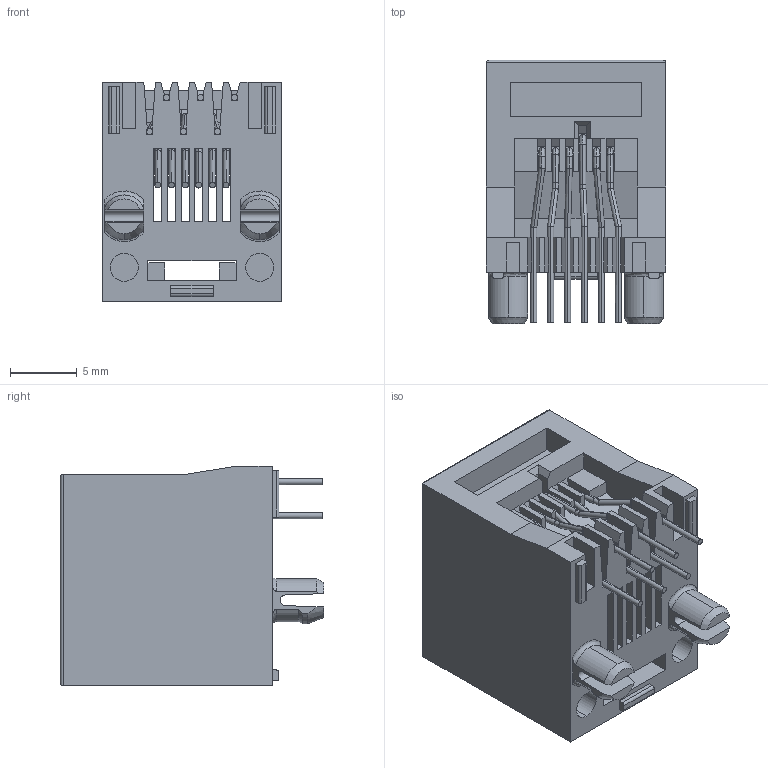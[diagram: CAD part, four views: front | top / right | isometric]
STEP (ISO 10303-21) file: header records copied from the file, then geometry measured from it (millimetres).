
FILE_DESCRIPTION (( 'STEP AP203' ), '1' );
FILE_NAME ('RJ24016661N00071.STEP', '2019-12-16T15:48:55', ( '' ), ( '' ), 'SwSTEP 2.0', 'SolidWorks 2016', '' );
FILE_SCHEMA (( 'CONFIG_CONTROL_DESIGN' ));
Length unit declared in the file: millimetre
Products named in the file (3): 24 Insulator_MBB; 24 Contacts_MBB; RJ24016661N00071
Assembly tree (2 placements, depth 2):
  RJ24016661N00071
    24 Insulator_MBB
    24 Contacts_MBB
Bounding box: 13.46 x 19.73 x 16.48 mm (x, y, z)
Volume: 1745.8 mm3; surface area: 2939.8 mm2
Topology: 7 solids, 7 shells, 450 faces, 1286 edges, 840 vertices
Faces by surface type: plane 262, cylinder 152, bspline 28, cone 8
Entity records: 15482 total; most frequent: CARTESIAN_POINT 3600, ORIENTED_EDGE 2572, DIRECTION 2273, EDGE_CURVE 1286, VECTOR 879, LINE 879, VERTEX_POINT 840, AXIS2_PLACEMENT_3D 697
